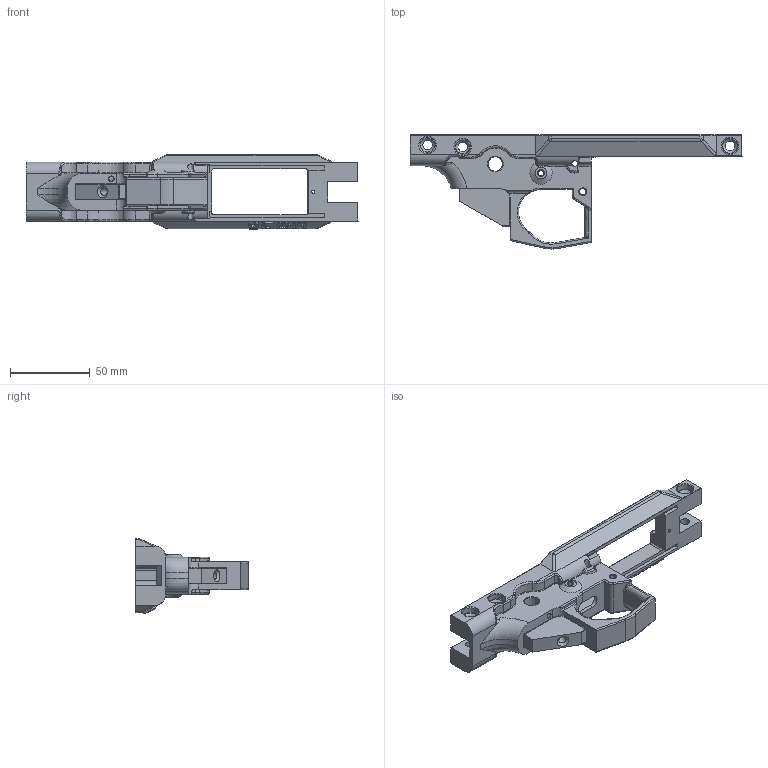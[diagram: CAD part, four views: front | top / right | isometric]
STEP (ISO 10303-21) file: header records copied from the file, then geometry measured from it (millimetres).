
FILE_DESCRIPTION(/* description */ (''),/* implementation_level */ '2;1');
FILE_NAME(/* name */ 'MOD6 Airsoft lower.stp',/* time_stamp */ '2020-10-18T11:24:34+03:00',/* author */ (''),/* organization */ (''),/* preprocessor_version */ 'ST-DEVELOPER v15.2',/* originating_system */ 'Autodesk Translator Framework v2.0.0.5431',/* authorisation */ '');
FILE_SCHEMA (('AUTOMOTIVE_DESIGN { 1 0 10303 214 3 1 1 }'));
Length unit declared in the file: centimetre
Products named in the file (1): MOD9 RETRACT FINAL ASSEMBLY MAGWELL FIXED 3 (production version)D
Bounding box: 207.56 x 71.26 x 46.46 mm (x, y, z)
Volume: 100925.6 mm3; surface area: 40424.6 mm2
Topology: 1 solids, 2 shells, 594 faces, 1594 edges, 993 vertices
Faces by surface type: plane 180, bspline 162, cylinder 157, torus 53, cone 36, sphere 6
Full cylindrical faces by diameter (mm): 2 x1, 3.175 x1, 3.469 x2, 3.5 x2, 4 x1, 4.605 x1, 6 x6, 9.025 x2, 10 x6
Entity records: 25581 total; most frequent: CARTESIAN_POINT 11993, ORIENTED_EDGE 3054, DIRECTION 2400, EDGE_CURVE 1526, VERTEX_POINT 981, AXIS2_PLACEMENT_3D 849, LINE 702, VECTOR 702
